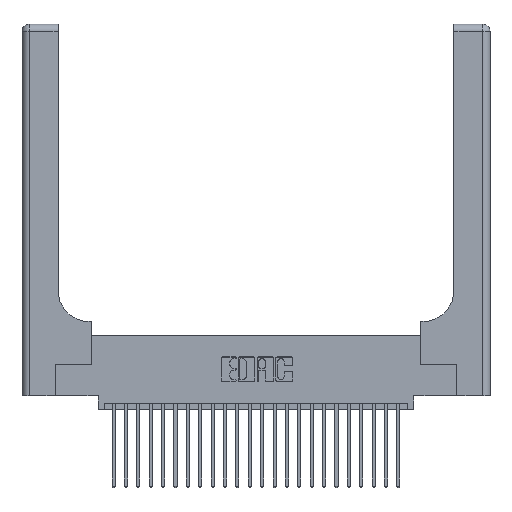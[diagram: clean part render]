
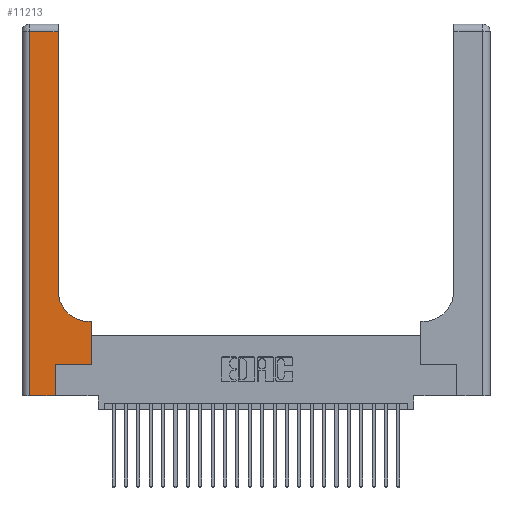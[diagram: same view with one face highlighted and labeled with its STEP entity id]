
A CAD part, top view. The second image highlights one B-rep face of the part: STEP entity #11213.
In plain terms, the highlighted planar face has unit normal (0, 0, 1).
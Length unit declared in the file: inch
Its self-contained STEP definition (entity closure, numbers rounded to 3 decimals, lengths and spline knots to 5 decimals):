
#378 = AXIS2_PLACEMENT_3D ( 'NONE', #11364, #13417, #1043 ) ;
#380 = EDGE_LOOP ( 'NONE', ( #12235, #565, #5429, #21221, #15405, #24991, #19586, #13479, #8013 ) ) ;
#508 = EDGE_CURVE ( 'NONE', #24467, #1116, #26085, .T. ) ;
#565 = ORIENTED_EDGE ( 'NONE', *, *, #6339, .T. ) ;
#1043 = DIRECTION ( 'NONE',  ( -1., 0., 0. ) ) ;
#1116 = VERTEX_POINT ( 'NONE', #5395 ) ;
#1267 = LINE ( 'NONE', #26381, #12281 ) ;
#1282 = FACE_OUTER_BOUND ( 'NONE', #380, .T. ) ;
#1480 = DIRECTION ( 'NONE',  ( 0., -1., 0. ) ) ;
#1982 = VERTEX_POINT ( 'NONE', #10725 ) ;
#2086 = CARTESIAN_POINT ( 'NONE',  ( 0.5585, 0.6, 0.37 ) ) ;
#2226 = VERTEX_POINT ( 'NONE', #7691 ) ;
#3366 = LINE ( 'NONE', #18083, #24548 ) ;
#3442 = VERTEX_POINT ( 'NONE', #25810 ) ;
#4050 = VERTEX_POINT ( 'NONE', #13264 ) ;
#4147 = CIRCLE ( 'NONE', #5199, 0.25 ) ;
#5199 = AXIS2_PLACEMENT_3D ( 'NONE', #7923, #22287, #10009 ) ;
#5395 = CARTESIAN_POINT ( 'NONE',  ( 0.5415, 0.6, 0.37 ) ) ;
#5429 = ORIENTED_EDGE ( 'NONE', *, *, #21327, .T. ) ;
#5627 = DIRECTION ( 'NONE',  ( 0., 1., 0. ) ) ;
#6007 = VECTOR ( 'NONE', #18919, 39.37008 ) ;
#6204 = EDGE_CURVE ( 'NONE', #24239, #1982, #1267, .T. ) ;
#6339 = EDGE_CURVE ( 'NONE', #4050, #2226, #14504, .T. ) ;
#7215 = VERTEX_POINT ( 'NONE', #26180 ) ;
#7247 = EDGE_CURVE ( 'NONE', #1116, #7495, #4147, .T. ) ;
#7495 = VERTEX_POINT ( 'NONE', #22967 ) ;
#7691 = CARTESIAN_POINT ( 'NONE',  ( 0.06, 2.94, 0.37 ) ) ;
#7876 = CARTESIAN_POINT ( 'NONE',  ( 0.269, 0., 0.37 ) ) ;
#7923 = CARTESIAN_POINT ( 'NONE',  ( 0.5415, 0.85, 0.37 ) ) ;
#8013 = ORIENTED_EDGE ( 'NONE', *, *, #7247, .T. ) ;
#8566 = DIRECTION ( 'NONE',  ( -1., 0., 0. ) ) ;
#9951 = VECTOR ( 'NONE', #5627, 39.37008 ) ;
#10009 = DIRECTION ( 'NONE',  ( 1., 0., 0. ) ) ;
#10428 = DIRECTION ( 'NONE',  ( -1., 0., 0. ) ) ;
#10486 = CARTESIAN_POINT ( 'NONE',  ( 0.2915, 0.6, 0.37 ) ) ;
#10559 = CARTESIAN_POINT ( 'NONE',  ( 0., 2.94, 0.37 ) ) ;
#10725 = CARTESIAN_POINT ( 'NONE',  ( 0.269, 0., 0.37 ) ) ;
#11213 = ADVANCED_FACE ( 'NONE', ( #1282 ), #23601, .F. ) ;
#11364 = CARTESIAN_POINT ( 'NONE',  ( 0., 3., 0.37 ) ) ;
#11496 = LINE ( 'NONE', #14773, #6007 ) ;
#12100 = DIRECTION ( 'NONE',  ( 1., 0., 0. ) ) ;
#12235 = ORIENTED_EDGE ( 'NONE', *, *, #15871, .T. ) ;
#12281 = VECTOR ( 'NONE', #12100, 39.37008 ) ;
#13001 = EDGE_CURVE ( 'NONE', #7215, #24467, #20246, .T. ) ;
#13264 = CARTESIAN_POINT ( 'NONE',  ( 0.2915, 2.94, 0.37 ) ) ;
#13417 = DIRECTION ( 'NONE',  ( 0., 0., -1. ) ) ;
#13479 = ORIENTED_EDGE ( 'NONE', *, *, #508, .T. ) ;
#14439 = LINE ( 'NONE', #7876, #25311 ) ;
#14504 = LINE ( 'NONE', #10559, #23440 ) ;
#14773 = CARTESIAN_POINT ( 'NONE',  ( 0.269, 0.25, 0.37 ) ) ;
#15405 = ORIENTED_EDGE ( 'NONE', *, *, #23745, .T. ) ;
#15479 = VECTOR ( 'NONE', #1480, 39.37008 ) ;
#15770 = CARTESIAN_POINT ( 'NONE',  ( 0.06, 0., 0.37 ) ) ;
#15871 = EDGE_CURVE ( 'NONE', #7495, #4050, #3366, .T. ) ;
#18083 = CARTESIAN_POINT ( 'NONE',  ( 0.2915, 3., 0.37 ) ) ;
#18919 = DIRECTION ( 'NONE',  ( 1., 0., 0. ) ) ;
#19586 = ORIENTED_EDGE ( 'NONE', *, *, #13001, .T. ) ;
#20061 = CARTESIAN_POINT ( 'NONE',  ( 0.5585, 0.25, 0.37 ) ) ;
#20216 = DIRECTION ( 'NONE',  ( 0., 1., 0. ) ) ;
#20246 = LINE ( 'NONE', #20061, #9951 ) ;
#21221 = ORIENTED_EDGE ( 'NONE', *, *, #6204, .T. ) ;
#21327 = EDGE_CURVE ( 'NONE', #2226, #24239, #26348, .T. ) ;
#21971 = VECTOR ( 'NONE', #10428, 39.37008 ) ;
#22287 = DIRECTION ( 'NONE',  ( 0., 0., -1. ) ) ;
#22967 = CARTESIAN_POINT ( 'NONE',  ( 0.2915, 0.85, 0.37 ) ) ;
#23440 = VECTOR ( 'NONE', #8566, 39.37008 ) ;
#23601 = PLANE ( 'NONE',  #378 ) ;
#23745 = EDGE_CURVE ( 'NONE', #1982, #3442, #14439, .T. ) ;
#24027 = CARTESIAN_POINT ( 'NONE',  ( 0.06, 3., 0.37 ) ) ;
#24239 = VERTEX_POINT ( 'NONE', #15770 ) ;
#24301 = DIRECTION ( 'NONE',  ( 0., 1., 0. ) ) ;
#24467 = VERTEX_POINT ( 'NONE', #2086 ) ;
#24548 = VECTOR ( 'NONE', #24301, 39.37008 ) ;
#24991 = ORIENTED_EDGE ( 'NONE', *, *, #26480, .T. ) ;
#25311 = VECTOR ( 'NONE', #20216, 39.37008 ) ;
#25810 = CARTESIAN_POINT ( 'NONE',  ( 0.269, 0.25, 0.37 ) ) ;
#26085 = LINE ( 'NONE', #10486, #21971 ) ;
#26180 = CARTESIAN_POINT ( 'NONE',  ( 0.5585, 0.25, 0.37 ) ) ;
#26348 = LINE ( 'NONE', #24027, #15479 ) ;
#26381 = CARTESIAN_POINT ( 'NONE',  ( 0., 0., 0.37 ) ) ;
#26480 = EDGE_CURVE ( 'NONE', #3442, #7215, #11496, .T. ) ;
